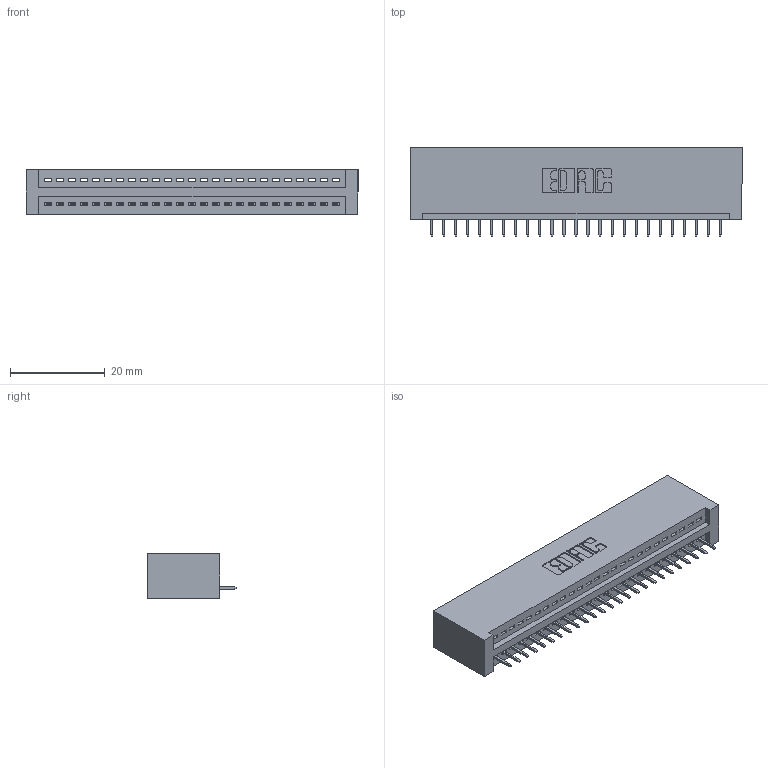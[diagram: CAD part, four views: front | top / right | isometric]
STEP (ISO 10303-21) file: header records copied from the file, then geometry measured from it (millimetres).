
FILE_DESCRIPTION (( 'STEP AP203' ), '1' );
FILE_NAME ('895-025-525-101.STEP', '2020-09-25T13:59:45', ( '' ), ( '' ), 'SwSTEP 2.0', 'SolidWorks 2020', '' );
FILE_SCHEMA (( 'CONFIG_CONTROL_DESIGN' ));
Length unit declared in the file: inch
Products named in the file (3): 895-025-525-101; 345-292-001_345-293-125; 845 Part_No Mounting Lugs
Assembly tree (26 placements, depth 2):
  895-025-525-101
    845 Part_No Mounting Lugs
    345-292-001_345-293-125  x25
Bounding box: 70.1 x 18.72 x 9.4 mm (x, y, z)
Volume: 7001.6 mm3; surface area: 8923.2 mm2
Topology: 26 solids, 26 shells, 1668 faces, 4817 edges, 3110 vertices
Faces by surface type: plane 1226, cylinder 442
Entity records: 20901 total; most frequent: CARTESIAN_POINT 3627, ORIENTED_EDGE 3586, DIRECTION 3187, EDGE_CURVE 1793, LINE 1573, VECTOR 1573, VERTEX_POINT 1190, AXIS2_PLACEMENT_3D 807
